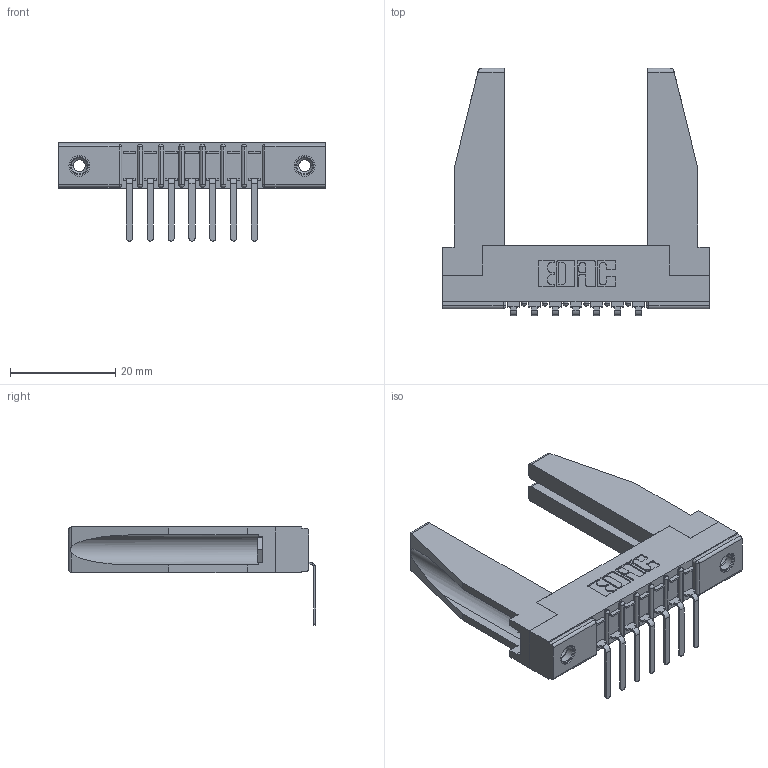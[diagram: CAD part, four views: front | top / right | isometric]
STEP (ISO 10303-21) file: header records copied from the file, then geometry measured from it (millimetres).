
FILE_DESCRIPTION (( 'STEP AP203' ), '1' );
FILE_NAME ('307-007-457-178.STEP', '2020-09-25T02:51:01', ( '' ), ( '' ), 'SwSTEP 2.0', 'SolidWorks 2020', '' );
FILE_SCHEMA (( 'CONFIG_CONTROL_DESIGN' ));
Length unit declared in the file: inch
Products named in the file (5): 307 Part_.156 Dia Mounting Holes; 307-290-002_557; 307-220-078; 307-007-457-178; 345-250-001_345-250-001-102
Assembly tree (12 placements, depth 2):
  307-007-457-178
    307 Part_.156 Dia Mounting Holes
    307-290-002_557  x7
    307-220-078  x2
    345-250-001_345-250-001-102  x2
Bounding box: 50.75 x 47.03 x 18.67 mm (x, y, z)
Volume: 7354.7 mm3; surface area: 9216 mm2
Topology: 12 solids, 12 shells, 802 faces, 2361 edges, 1542 vertices
Faces by surface type: plane 483, cylinder 287, sphere 16, cone 12, torus 4
Entity records: 13609 total; most frequent: CARTESIAN_POINT 2290, ORIENTED_EDGE 2236, DIRECTION 2198, EDGE_CURVE 1118, LINE 842, VECTOR 842, VERTEX_POINT 728, AXIS2_PLACEMENT_3D 678
